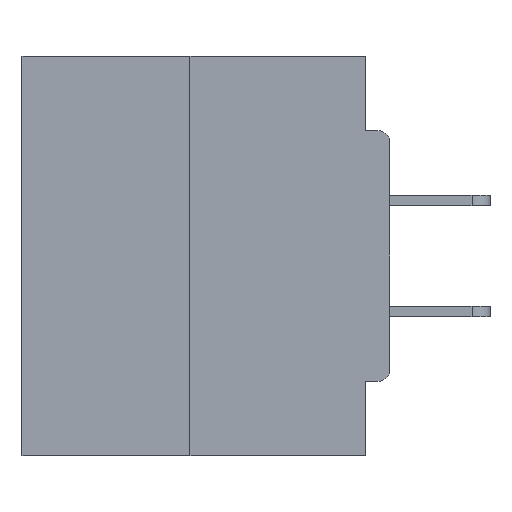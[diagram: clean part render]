
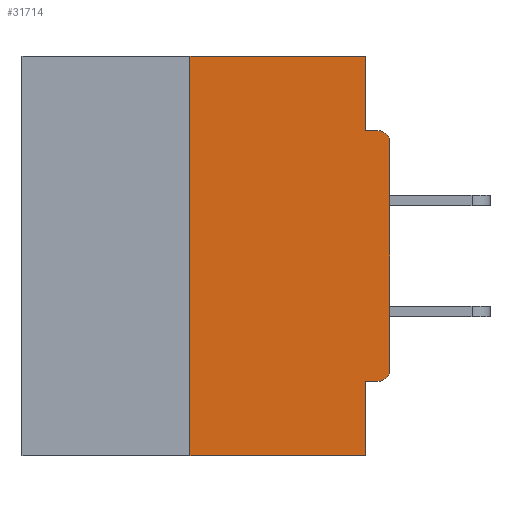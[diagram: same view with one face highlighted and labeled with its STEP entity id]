
A CAD part, left-side view. The second image highlights one B-rep face of the part: STEP entity #31714.
In plain terms, the highlighted planar face has unit normal (-1, 0, 0).
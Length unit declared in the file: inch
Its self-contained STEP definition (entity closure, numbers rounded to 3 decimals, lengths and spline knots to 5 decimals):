
#335 = VECTOR ( 'NONE', #27978, 39.37008 ) ;
#360 = CARTESIAN_POINT ( 'NONE',  ( 0., 0.031, -0.0935 ) ) ;
#1103 = LINE ( 'NONE', #3321, #335 ) ;
#1473 = ORIENTED_EDGE ( 'NONE', *, *, #4604, .T. ) ;
#2052 = VECTOR ( 'NONE', #16595, 39.37008 ) ;
#2205 = ORIENTED_EDGE ( 'NONE', *, *, #25174, .F. ) ;
#2488 = VERTEX_POINT ( 'NONE', #31751 ) ;
#3321 = CARTESIAN_POINT ( 'NONE',  ( 0., 0.031, -0.5 ) ) ;
#3594 = LINE ( 'NONE', #12010, #18851 ) ;
#3671 = DIRECTION ( 'NONE',  ( 0., -1., 0. ) ) ;
#3945 = CARTESIAN_POINT ( 'NONE',  ( 0., 0.25, 0. ) ) ;
#3992 = EDGE_CURVE ( 'NONE', #24850, #11027, #27406, .T. ) ;
#4068 = CARTESIAN_POINT ( 'NONE',  ( 0., 0.25, -0.5 ) ) ;
#4356 = EDGE_CURVE ( 'NONE', #24850, #29373, #12133, .T. ) ;
#4514 = DIRECTION ( 'NONE',  ( 0., 0., -1. ) ) ;
#4604 = EDGE_CURVE ( 'NONE', #11428, #23808, #8617, .T. ) ;
#5265 = CARTESIAN_POINT ( 'NONE',  ( 0., 0.031, 0. ) ) ;
#5275 = CARTESIAN_POINT ( 'NONE',  ( 0., 0.015, -0.0935 ) ) ;
#5448 = CIRCLE ( 'NONE', #21343, 0.015 ) ;
#7046 = EDGE_CURVE ( 'NONE', #24317, #29373, #1103, .T. ) ;
#7424 = VECTOR ( 'NONE', #16514, 39.37008 ) ;
#7473 = EDGE_CURVE ( 'NONE', #2488, #24317, #29201, .T. ) ;
#7786 = DIRECTION ( 'NONE',  ( 0., 0., -1. ) ) ;
#7891 = DIRECTION ( 'NONE',  ( -1., 0., 0. ) ) ;
#8385 = VERTEX_POINT ( 'NONE', #5275 ) ;
#8617 = LINE ( 'NONE', #19370, #2052 ) ;
#9246 = VERTEX_POINT ( 'NONE', #360 ) ;
#9797 = CARTESIAN_POINT ( 'NONE',  ( 0., 0., -0.1085 ) ) ;
#10228 = DIRECTION ( 'NONE',  ( 0., 0., -1. ) ) ;
#10814 = ORIENTED_EDGE ( 'NONE', *, *, #18813, .F. ) ;
#11013 = CARTESIAN_POINT ( 'NONE',  ( 0., 0., -0.0935 ) ) ;
#11027 = VERTEX_POINT ( 'NONE', #15679 ) ;
#11179 = VECTOR ( 'NONE', #27693, 39.37008 ) ;
#11342 = EDGE_CURVE ( 'NONE', #23808, #8385, #5448, .T. ) ;
#11428 = VERTEX_POINT ( 'NONE', #23135 ) ;
#12010 = CARTESIAN_POINT ( 'NONE',  ( 0., 0.031, 0. ) ) ;
#12133 = LINE ( 'NONE', #26504, #13657 ) ;
#12194 = VECTOR ( 'NONE', #13538, 39.37008 ) ;
#13032 = CARTESIAN_POINT ( 'NONE',  ( 0., 0.46, 0. ) ) ;
#13347 = PLANE ( 'NONE',  #22597 ) ;
#13367 = LINE ( 'NONE', #11013, #12194 ) ;
#13538 = DIRECTION ( 'NONE',  ( 0., -1., 0. ) ) ;
#13657 = VECTOR ( 'NONE', #18799, 39.37008 ) ;
#13906 = AXIS2_PLACEMENT_3D ( 'NONE', #20200, #7891, #7786 ) ;
#13930 = VERTEX_POINT ( 'NONE', #5265 ) ;
#15534 = EDGE_CURVE ( 'NONE', #9246, #8385, #13367, .T. ) ;
#15679 = CARTESIAN_POINT ( 'NONE',  ( 0., 0.25, 0. ) ) ;
#16514 = DIRECTION ( 'NONE',  ( 0., 0., 1. ) ) ;
#16595 = DIRECTION ( 'NONE',  ( 0., 0., 1. ) ) ;
#18391 = EDGE_CURVE ( 'NONE', #2488, #11428, #31712, .T. ) ;
#18799 = DIRECTION ( 'NONE',  ( 0., -1., 0. ) ) ;
#18813 = EDGE_CURVE ( 'NONE', #13930, #9246, #3594, .T. ) ;
#18851 = VECTOR ( 'NONE', #4514, 39.37008 ) ;
#19370 = CARTESIAN_POINT ( 'NONE',  ( 0., 0., 0. ) ) ;
#19744 = LINE ( 'NONE', #30941, #24023 ) ;
#20200 = CARTESIAN_POINT ( 'NONE',  ( 0., 0.015, -0.3915 ) ) ;
#20958 = DIRECTION ( 'NONE',  ( 1., 0., 0. ) ) ;
#21013 = ORIENTED_EDGE ( 'NONE', *, *, #15534, .F. ) ;
#21237 = ORIENTED_EDGE ( 'NONE', *, *, #7473, .F. ) ;
#21343 = AXIS2_PLACEMENT_3D ( 'NONE', #22708, #30090, #10228 ) ;
#22130 = CARTESIAN_POINT ( 'NONE',  ( 0., 0.031, -0.5 ) ) ;
#22439 = ORIENTED_EDGE ( 'NONE', *, *, #3992, .F. ) ;
#22597 = AXIS2_PLACEMENT_3D ( 'NONE', #13032, #20958, #30927 ) ;
#22620 = CARTESIAN_POINT ( 'NONE',  ( 0., 0.031, -0.4065 ) ) ;
#22708 = CARTESIAN_POINT ( 'NONE',  ( 0., 0.015, -0.1085 ) ) ;
#23135 = CARTESIAN_POINT ( 'NONE',  ( 0., 0., -0.3915 ) ) ;
#23808 = VERTEX_POINT ( 'NONE', #9797 ) ;
#24023 = VECTOR ( 'NONE', #3671, 39.37008 ) ;
#24267 = ORIENTED_EDGE ( 'NONE', *, *, #11342, .T. ) ;
#24317 = VERTEX_POINT ( 'NONE', #22620 ) ;
#24850 = VERTEX_POINT ( 'NONE', #4068 ) ;
#25174 = EDGE_CURVE ( 'NONE', #11027, #13930, #19744, .T. ) ;
#25860 = CARTESIAN_POINT ( 'NONE',  ( 0., 0., -0.4065 ) ) ;
#26504 = CARTESIAN_POINT ( 'NONE',  ( 0., 0.46, -0.5 ) ) ;
#27406 = LINE ( 'NONE', #3945, #7424 ) ;
#27664 = ORIENTED_EDGE ( 'NONE', *, *, #4356, .T. ) ;
#27693 = DIRECTION ( 'NONE',  ( 0., 1., 0. ) ) ;
#27978 = DIRECTION ( 'NONE',  ( 0., 0., -1. ) ) ;
#29201 = LINE ( 'NONE', #25860, #11179 ) ;
#29373 = VERTEX_POINT ( 'NONE', #22130 ) ;
#29663 = FACE_OUTER_BOUND ( 'NONE', #31612, .T. ) ;
#30090 = DIRECTION ( 'NONE',  ( -1., 0., 0. ) ) ;
#30510 = ORIENTED_EDGE ( 'NONE', *, *, #7046, .F. ) ;
#30845 = ORIENTED_EDGE ( 'NONE', *, *, #18391, .T. ) ;
#30927 = DIRECTION ( 'NONE',  ( 0., 0., -1. ) ) ;
#30941 = CARTESIAN_POINT ( 'NONE',  ( 0., 0.46, 0. ) ) ;
#31612 = EDGE_LOOP ( 'NONE', ( #2205, #22439, #27664, #30510, #21237, #30845, #1473, #24267, #21013, #10814 ) ) ;
#31712 = CIRCLE ( 'NONE', #13906, 0.015 ) ;
#31714 = ADVANCED_FACE ( 'NONE', ( #29663 ), #13347, .F. ) ;
#31751 = CARTESIAN_POINT ( 'NONE',  ( 0., 0.015, -0.4065 ) ) ;
